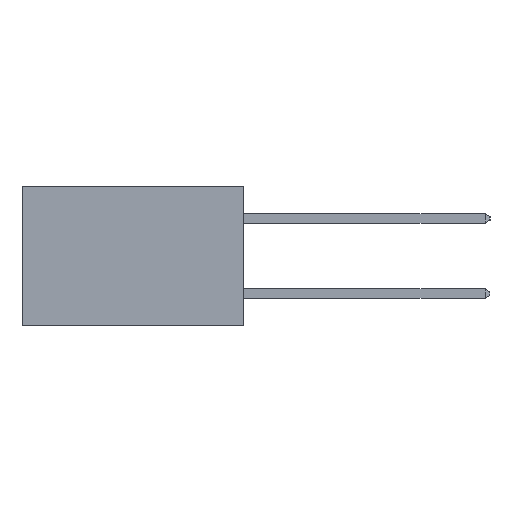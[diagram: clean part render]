
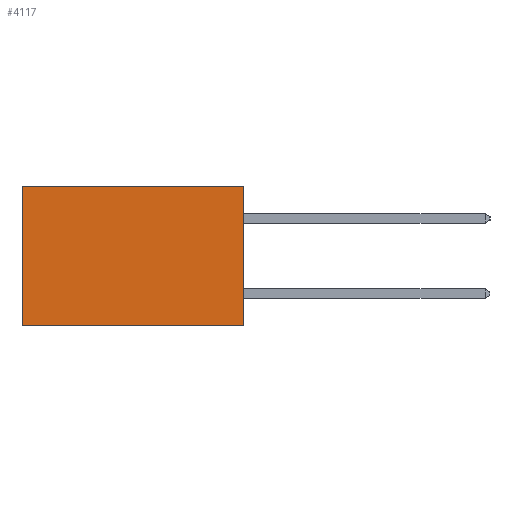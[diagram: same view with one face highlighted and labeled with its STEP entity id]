
A CAD part, left-side view. The second image highlights one B-rep face of the part: STEP entity #4117.
In plain terms, the highlighted planar face has unit normal (-1, 0, 0).
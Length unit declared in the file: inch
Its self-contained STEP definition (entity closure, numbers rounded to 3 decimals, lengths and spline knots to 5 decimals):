
#64 = VECTOR ( 'NONE', #6779, 39.37008 ) ;
#1346 = VECTOR ( 'NONE', #3020, 39.37008 ) ;
#1350 = CARTESIAN_POINT ( 'NONE',  ( 0.277, 0.59, -0.37 ) ) ;
#2093 = VERTEX_POINT ( 'NONE', #16374 ) ;
#3020 = DIRECTION ( 'NONE',  ( 0., 0., -1. ) ) ;
#3291 = PLANE ( 'NONE',  #19509 ) ;
#3448 = CARTESIAN_POINT ( 'NONE',  ( 0.277, 0.59, 0. ) ) ;
#3697 = CARTESIAN_POINT ( 'NONE',  ( 0.277, 0., -0.37 ) ) ;
#4113 = EDGE_LOOP ( 'NONE', ( #15831, #16311, #8485, #12734 ) ) ;
#4117 = ADVANCED_FACE ( 'NONE', ( #14728 ), #3291, .F. ) ;
#4329 = EDGE_CURVE ( 'NONE', #5934, #18112, #10306, .T. ) ;
#4375 = CARTESIAN_POINT ( 'NONE',  ( 0.277, 0., -0.37 ) ) ;
#5127 = CARTESIAN_POINT ( 'NONE',  ( 0.277, 0., 0. ) ) ;
#5823 = EDGE_CURVE ( 'NONE', #2093, #5934, #8760, .T. ) ;
#5934 = VERTEX_POINT ( 'NONE', #12432 ) ;
#6038 = VECTOR ( 'NONE', #6580, 39.37008 ) ;
#6580 = DIRECTION ( 'NONE',  ( 0., 1., 0. ) ) ;
#6779 = DIRECTION ( 'NONE',  ( 0., 1., 0. ) ) ;
#8485 = ORIENTED_EDGE ( 'NONE', *, *, #5823, .F. ) ;
#8760 = LINE ( 'NONE', #15465, #16568 ) ;
#9969 = LINE ( 'NONE', #1350, #1346 ) ;
#10306 = LINE ( 'NONE', #3697, #6038 ) ;
#10578 = EDGE_CURVE ( 'NONE', #18167, #18112, #9969, .T. ) ;
#10943 = CARTESIAN_POINT ( 'NONE',  ( 0.277, 0.59, -0.37 ) ) ;
#12432 = CARTESIAN_POINT ( 'NONE',  ( 0.277, 0., -0.37 ) ) ;
#12734 = ORIENTED_EDGE ( 'NONE', *, *, #14915, .T. ) ;
#14728 = FACE_OUTER_BOUND ( 'NONE', #4113, .T. ) ;
#14915 = EDGE_CURVE ( 'NONE', #2093, #18167, #18036, .T. ) ;
#15465 = CARTESIAN_POINT ( 'NONE',  ( 0.277, 0., -0.37 ) ) ;
#15831 = ORIENTED_EDGE ( 'NONE', *, *, #10578, .T. ) ;
#15843 = DIRECTION ( 'NONE',  ( 0., 0., -1. ) ) ;
#16311 = ORIENTED_EDGE ( 'NONE', *, *, #4329, .F. ) ;
#16374 = CARTESIAN_POINT ( 'NONE',  ( 0.277, 0., 0. ) ) ;
#16568 = VECTOR ( 'NONE', #15843, 39.37008 ) ;
#18036 = LINE ( 'NONE', #5127, #64 ) ;
#18112 = VERTEX_POINT ( 'NONE', #10943 ) ;
#18167 = VERTEX_POINT ( 'NONE', #3448 ) ;
#19037 = DIRECTION ( 'NONE',  ( 0., 0., -1. ) ) ;
#19386 = DIRECTION ( 'NONE',  ( 1., 0., 0. ) ) ;
#19509 = AXIS2_PLACEMENT_3D ( 'NONE', #4375, #19386, #19037 ) ;
